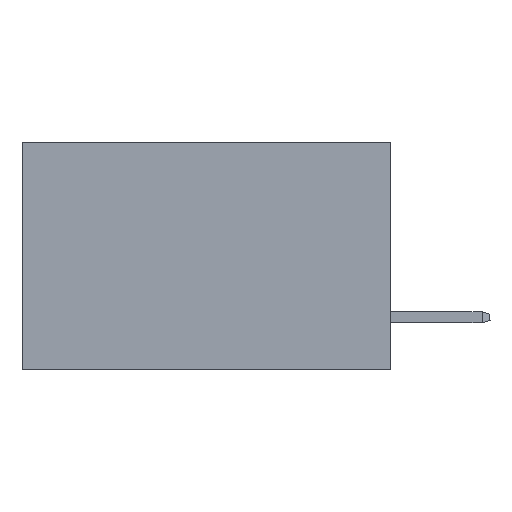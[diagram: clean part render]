
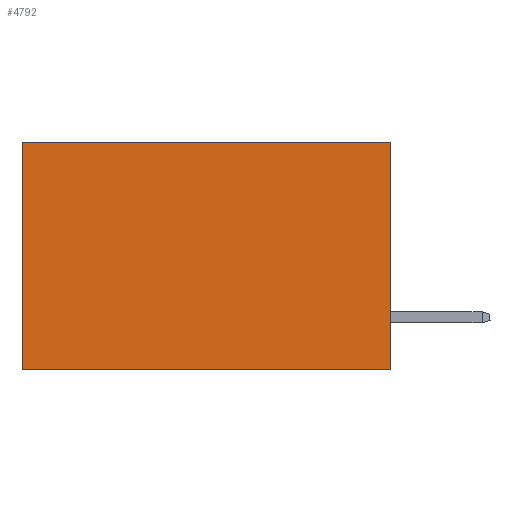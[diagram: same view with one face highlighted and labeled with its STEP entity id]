
A CAD part, left-side view. The second image highlights one B-rep face of the part: STEP entity #4792.
In plain terms, the highlighted planar face has unit normal (-1, 0, 0).
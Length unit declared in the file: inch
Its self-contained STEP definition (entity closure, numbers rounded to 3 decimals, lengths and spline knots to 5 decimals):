
#228 = DIRECTION ( 'NONE',  ( 0., 0., -1. ) ) ;
#847 = DIRECTION ( 'NONE',  ( 0., 1., 0. ) ) ;
#1450 = LINE ( 'NONE', #28673, #31999 ) ;
#2801 = CARTESIAN_POINT ( 'NONE',  ( 0.2875, 0., 0. ) ) ;
#3891 = PLANE ( 'NONE',  #26883 ) ;
#4461 = FACE_OUTER_BOUND ( 'NONE', #30041, .T. ) ;
#4792 = ADVANCED_FACE ( 'NONE', ( #4461 ), #3891, .F. ) ;
#6130 = DIRECTION ( 'NONE',  ( 1., 0., 0. ) ) ;
#6897 = EDGE_CURVE ( 'NONE', #18865, #9165, #1450, .T. ) ;
#7482 = LINE ( 'NONE', #29987, #14673 ) ;
#7892 = VERTEX_POINT ( 'NONE', #10547 ) ;
#7962 = DIRECTION ( 'NONE',  ( 0., 0., -1. ) ) ;
#8441 = EDGE_CURVE ( 'NONE', #7892, #33095, #7482, .T. ) ;
#9165 = VERTEX_POINT ( 'NONE', #18522 ) ;
#10547 = CARTESIAN_POINT ( 'NONE',  ( 0.2875, 0., -0.37 ) ) ;
#11119 = VECTOR ( 'NONE', #7962, 39.37008 ) ;
#12183 = EDGE_CURVE ( 'NONE', #18865, #7892, #24824, .T. ) ;
#13008 = CARTESIAN_POINT ( 'NONE',  ( 0.2875, 0.6, 0. ) ) ;
#13403 = CARTESIAN_POINT ( 'NONE',  ( 0.2875, 0.6, -0.37 ) ) ;
#14596 = CARTESIAN_POINT ( 'NONE',  ( 0.2875, 0., 0. ) ) ;
#14623 = DIRECTION ( 'NONE',  ( 0., 1., 0. ) ) ;
#14673 = VECTOR ( 'NONE', #14623, 39.37008 ) ;
#18522 = CARTESIAN_POINT ( 'NONE',  ( 0.2875, 0.6, 0. ) ) ;
#18591 = ORIENTED_EDGE ( 'NONE', *, *, #8441, .F. ) ;
#18865 = VERTEX_POINT ( 'NONE', #14596 ) ;
#19931 = ORIENTED_EDGE ( 'NONE', *, *, #6897, .T. ) ;
#23425 = CARTESIAN_POINT ( 'NONE',  ( 0.2875, 0., 0. ) ) ;
#24824 = LINE ( 'NONE', #23425, #11119 ) ;
#26883 = AXIS2_PLACEMENT_3D ( 'NONE', #2801, #6130, #30121 ) ;
#27129 = ORIENTED_EDGE ( 'NONE', *, *, #12183, .F. ) ;
#28673 = CARTESIAN_POINT ( 'NONE',  ( 0.2875, 0., 0. ) ) ;
#28985 = ORIENTED_EDGE ( 'NONE', *, *, #30427, .T. ) ;
#29987 = CARTESIAN_POINT ( 'NONE',  ( 0.2875, 0., -0.37 ) ) ;
#30041 = EDGE_LOOP ( 'NONE', ( #28985, #18591, #27129, #19931 ) ) ;
#30121 = DIRECTION ( 'NONE',  ( 0., 0., -1. ) ) ;
#30149 = VECTOR ( 'NONE', #228, 39.37008 ) ;
#30427 = EDGE_CURVE ( 'NONE', #9165, #33095, #31332, .T. ) ;
#31332 = LINE ( 'NONE', #13008, #30149 ) ;
#31999 = VECTOR ( 'NONE', #847, 39.37008 ) ;
#33095 = VERTEX_POINT ( 'NONE', #13403 ) ;
